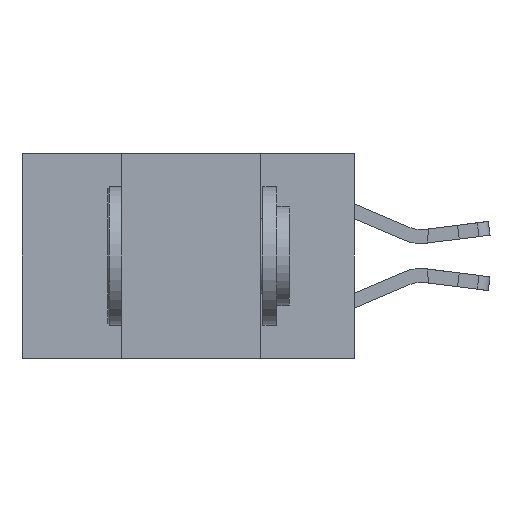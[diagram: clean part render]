
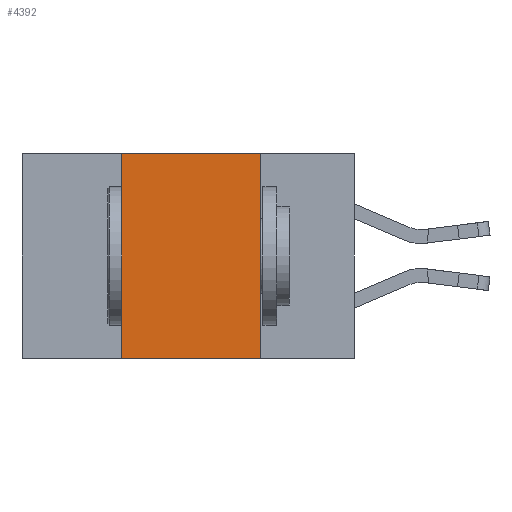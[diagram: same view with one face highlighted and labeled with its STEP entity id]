
A CAD part, left-side view. The second image highlights one B-rep face of the part: STEP entity #4392.
In plain terms, the highlighted planar face has unit normal (-1, 0, 0).
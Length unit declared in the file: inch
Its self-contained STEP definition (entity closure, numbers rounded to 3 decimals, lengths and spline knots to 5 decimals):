
#291 = LINE ( 'NONE', #7860, #16427 ) ;
#850 = ORIENTED_EDGE ( 'NONE', *, *, #8638, .F. ) ;
#1276 = VERTEX_POINT ( 'NONE', #4157 ) ;
#2658 = CARTESIAN_POINT ( 'NONE',  ( 0., 0.42, -0.37 ) ) ;
#3402 = ORIENTED_EDGE ( 'NONE', *, *, #7395, .F. ) ;
#4030 = DIRECTION ( 'NONE',  ( 0., 0., -1. ) ) ;
#4157 = CARTESIAN_POINT ( 'NONE',  ( 0., 0.17, 0. ) ) ;
#4392 = ADVANCED_FACE ( 'NONE', ( #11520 ), #11810, .F. ) ;
#4799 = VERTEX_POINT ( 'NONE', #13062 ) ;
#4908 = EDGE_CURVE ( 'NONE', #4799, #12015, #6440, .T. ) ;
#5067 = DIRECTION ( 'NONE',  ( 0., -1., 0. ) ) ;
#5115 = LINE ( 'NONE', #2658, #18666 ) ;
#5780 = CARTESIAN_POINT ( 'NONE',  ( 0., 0.42, 0. ) ) ;
#6378 = DIRECTION ( 'NONE',  ( 0., -1., 0. ) ) ;
#6410 = VECTOR ( 'NONE', #5067, 39.37008 ) ;
#6440 = LINE ( 'NONE', #15511, #6410 ) ;
#6721 = CARTESIAN_POINT ( 'NONE',  ( 0., 0.17, -0.37 ) ) ;
#7072 = VECTOR ( 'NONE', #15484, 39.37008 ) ;
#7361 = DIRECTION ( 'NONE',  ( 0., 0., 1. ) ) ;
#7395 = EDGE_CURVE ( 'NONE', #4799, #9966, #5115, .T. ) ;
#7860 = CARTESIAN_POINT ( 'NONE',  ( 0., 0.6, 0. ) ) ;
#7994 = CARTESIAN_POINT ( 'NONE',  ( 0., 0.17, -0.37 ) ) ;
#8638 = EDGE_CURVE ( 'NONE', #1276, #12015, #17155, .T. ) ;
#8765 = CARTESIAN_POINT ( 'NONE',  ( 0., 0.6, 0. ) ) ;
#9424 = ORIENTED_EDGE ( 'NONE', *, *, #4908, .T. ) ;
#9966 = VERTEX_POINT ( 'NONE', #5780 ) ;
#11520 = FACE_OUTER_BOUND ( 'NONE', #12084, .T. ) ;
#11810 = PLANE ( 'NONE',  #17090 ) ;
#12015 = VERTEX_POINT ( 'NONE', #6721 ) ;
#12084 = EDGE_LOOP ( 'NONE', ( #850, #16102, #3402, #9424 ) ) ;
#13062 = CARTESIAN_POINT ( 'NONE',  ( 0., 0.42, -0.37 ) ) ;
#15149 = EDGE_CURVE ( 'NONE', #9966, #1276, #291, .T. ) ;
#15484 = DIRECTION ( 'NONE',  ( 0., 0., -1. ) ) ;
#15511 = CARTESIAN_POINT ( 'NONE',  ( 0., 0.6, -0.37 ) ) ;
#16102 = ORIENTED_EDGE ( 'NONE', *, *, #15149, .F. ) ;
#16427 = VECTOR ( 'NONE', #6378, 39.37008 ) ;
#17090 = AXIS2_PLACEMENT_3D ( 'NONE', #8765, #17793, #4030 ) ;
#17155 = LINE ( 'NONE', #7994, #7072 ) ;
#17793 = DIRECTION ( 'NONE',  ( 1., 0., 0. ) ) ;
#18666 = VECTOR ( 'NONE', #7361, 39.37008 ) ;
